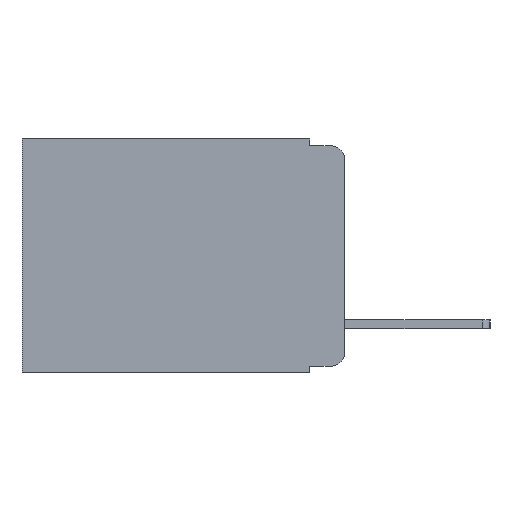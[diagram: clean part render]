
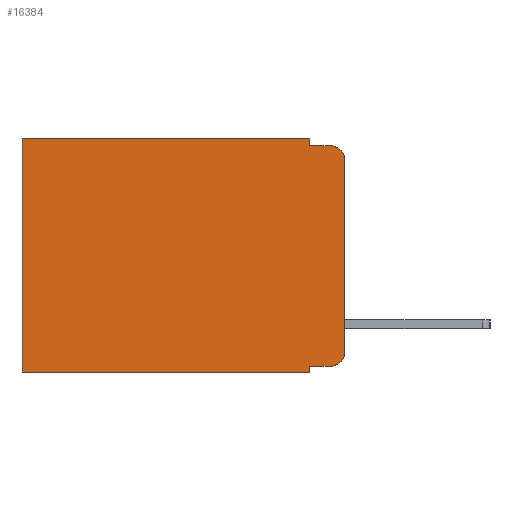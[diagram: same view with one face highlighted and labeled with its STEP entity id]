
A CAD part, left-side view. The second image highlights one B-rep face of the part: STEP entity #16384.
In plain terms, the highlighted planar face has unit normal (-1, 0, 0).
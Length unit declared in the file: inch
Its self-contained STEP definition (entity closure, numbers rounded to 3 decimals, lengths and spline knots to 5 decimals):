
#145 = ORIENTED_EDGE ( 'NONE', *, *, #16762, .F. ) ;
#662 = EDGE_CURVE ( 'NONE', #12113, #1314, #10611, .T. ) ;
#740 = CARTESIAN_POINT ( 'NONE',  ( 0.298, 0.051, -0.333 ) ) ;
#1314 = VERTEX_POINT ( 'NONE', #7506 ) ;
#1507 = DIRECTION ( 'NONE',  ( 0., 0., -1. ) ) ;
#2196 = CARTESIAN_POINT ( 'NONE',  ( 0.298, 0., -0.313 ) ) ;
#2331 = CIRCLE ( 'NONE', #8159, 0.02 ) ;
#2427 = VECTOR ( 'NONE', #5516, 39.37008 ) ;
#2864 = EDGE_CURVE ( 'NONE', #17752, #1314, #19845, .T. ) ;
#2885 = LINE ( 'NONE', #9695, #7057 ) ;
#3372 = AXIS2_PLACEMENT_3D ( 'NONE', #18085, #18155, #8942 ) ;
#3554 = LINE ( 'NONE', #16618, #7681 ) ;
#4242 = VECTOR ( 'NONE', #14819, 39.37008 ) ;
#4552 = VERTEX_POINT ( 'NONE', #19593 ) ;
#4815 = VERTEX_POINT ( 'NONE', #13018 ) ;
#5064 = DIRECTION ( 'NONE',  ( 0., 0., -1. ) ) ;
#5355 = VERTEX_POINT ( 'NONE', #2196 ) ;
#5516 = DIRECTION ( 'NONE',  ( 0., 1., 0. ) ) ;
#5737 = DIRECTION ( 'NONE',  ( 0., 0., -1. ) ) ;
#5811 = DIRECTION ( 'NONE',  ( 0., -1., 0. ) ) ;
#5813 = DIRECTION ( 'NONE',  ( 0., -1., 0. ) ) ;
#6029 = EDGE_CURVE ( 'NONE', #17752, #5355, #16909, .T. ) ;
#7057 = VECTOR ( 'NONE', #18810, 39.37008 ) ;
#7402 = PLANE ( 'NONE',  #3372 ) ;
#7426 = CARTESIAN_POINT ( 'NONE',  ( 0.298, 0.051, 0. ) ) ;
#7506 = CARTESIAN_POINT ( 'NONE',  ( 0.298, 0.02, -0.01 ) ) ;
#7681 = VECTOR ( 'NONE', #5813, 39.37008 ) ;
#8159 = AXIS2_PLACEMENT_3D ( 'NONE', #20023, #10915, #1507 ) ;
#8546 = CARTESIAN_POINT ( 'NONE',  ( 0.298, 0., -0.343 ) ) ;
#8942 = DIRECTION ( 'NONE',  ( 0., 0., -1. ) ) ;
#9107 = CARTESIAN_POINT ( 'NONE',  ( 0.298, 0.051, -0.01 ) ) ;
#9144 = CARTESIAN_POINT ( 'NONE',  ( 0.298, 0.051, -0.01 ) ) ;
#9329 = LINE ( 'NONE', #17887, #4242 ) ;
#9364 = ORIENTED_EDGE ( 'NONE', *, *, #14698, .T. ) ;
#9695 = CARTESIAN_POINT ( 'NONE',  ( 0.298, 0., 0. ) ) ;
#10480 = AXIS2_PLACEMENT_3D ( 'NONE', #18902, #11712, #13078 ) ;
#10611 = LINE ( 'NONE', #9107, #18732 ) ;
#10915 = DIRECTION ( 'NONE',  ( -1., 0., 0. ) ) ;
#11010 = VERTEX_POINT ( 'NONE', #13033 ) ;
#11119 = LINE ( 'NONE', #15153, #12104 ) ;
#11564 = FACE_OUTER_BOUND ( 'NONE', #17800, .T. ) ;
#11712 = DIRECTION ( 'NONE',  ( -1., 0., 0. ) ) ;
#11874 = EDGE_CURVE ( 'NONE', #11010, #4815, #14856, .T. ) ;
#11888 = ORIENTED_EDGE ( 'NONE', *, *, #2864, .T. ) ;
#12104 = VECTOR ( 'NONE', #16704, 39.37008 ) ;
#12113 = VERTEX_POINT ( 'NONE', #9144 ) ;
#12821 = CARTESIAN_POINT ( 'NONE',  ( 0.298, 0., 0. ) ) ;
#12844 = VECTOR ( 'NONE', #5064, 39.37008 ) ;
#13018 = CARTESIAN_POINT ( 'NONE',  ( 0.298, 0.473, -0.343 ) ) ;
#13033 = CARTESIAN_POINT ( 'NONE',  ( 0.298, 0.051, -0.343 ) ) ;
#13078 = DIRECTION ( 'NONE',  ( 0., 0., -1. ) ) ;
#13600 = ORIENTED_EDGE ( 'NONE', *, *, #18745, .T. ) ;
#13805 = ORIENTED_EDGE ( 'NONE', *, *, #14224, .T. ) ;
#14224 = EDGE_CURVE ( 'NONE', #17528, #16051, #2885, .T. ) ;
#14271 = CARTESIAN_POINT ( 'NONE',  ( 0.298, 0., -0.03 ) ) ;
#14698 = EDGE_CURVE ( 'NONE', #4552, #5355, #2331, .T. ) ;
#14819 = DIRECTION ( 'NONE',  ( 0., 0., -1. ) ) ;
#14856 = LINE ( 'NONE', #8546, #2427 ) ;
#15093 = ORIENTED_EDGE ( 'NONE', *, *, #11874, .F. ) ;
#15153 = CARTESIAN_POINT ( 'NONE',  ( 0.298, 0.473, 0. ) ) ;
#15751 = EDGE_CURVE ( 'NONE', #16275, #4552, #3554, .T. ) ;
#15918 = VECTOR ( 'NONE', #5737, 39.37008 ) ;
#16051 = VERTEX_POINT ( 'NONE', #17235 ) ;
#16275 = VERTEX_POINT ( 'NONE', #740 ) ;
#16383 = LINE ( 'NONE', #18110, #15918 ) ;
#16384 = ADVANCED_FACE ( 'NONE', ( #11564 ), #7402, .F. ) ;
#16618 = CARTESIAN_POINT ( 'NONE',  ( 0.298, 0.051, -0.333 ) ) ;
#16704 = DIRECTION ( 'NONE',  ( 0., 0., -1. ) ) ;
#16762 = EDGE_CURVE ( 'NONE', #16275, #11010, #9329, .T. ) ;
#16909 = LINE ( 'NONE', #12821, #12844 ) ;
#17235 = CARTESIAN_POINT ( 'NONE',  ( 0.298, 0.473, 0. ) ) ;
#17288 = ORIENTED_EDGE ( 'NONE', *, *, #6029, .F. ) ;
#17528 = VERTEX_POINT ( 'NONE', #7426 ) ;
#17752 = VERTEX_POINT ( 'NONE', #14271 ) ;
#17800 = EDGE_LOOP ( 'NONE', ( #17288, #11888, #18341, #18272, #13805, #13600, #15093, #145, #18285, #9364 ) ) ;
#17887 = CARTESIAN_POINT ( 'NONE',  ( 0.298, 0.051, 0. ) ) ;
#18085 = CARTESIAN_POINT ( 'NONE',  ( 0.298, 0., 0. ) ) ;
#18110 = CARTESIAN_POINT ( 'NONE',  ( 0.298, 0.051, 0. ) ) ;
#18155 = DIRECTION ( 'NONE',  ( 1., 0., 0. ) ) ;
#18272 = ORIENTED_EDGE ( 'NONE', *, *, #19746, .F. ) ;
#18285 = ORIENTED_EDGE ( 'NONE', *, *, #15751, .T. ) ;
#18341 = ORIENTED_EDGE ( 'NONE', *, *, #662, .F. ) ;
#18732 = VECTOR ( 'NONE', #5811, 39.37008 ) ;
#18745 = EDGE_CURVE ( 'NONE', #16051, #4815, #11119, .T. ) ;
#18810 = DIRECTION ( 'NONE',  ( 0., 1., 0. ) ) ;
#18902 = CARTESIAN_POINT ( 'NONE',  ( 0.298, 0.02, -0.03 ) ) ;
#19593 = CARTESIAN_POINT ( 'NONE',  ( 0.298, 0.02, -0.333 ) ) ;
#19746 = EDGE_CURVE ( 'NONE', #17528, #12113, #16383, .T. ) ;
#19845 = CIRCLE ( 'NONE', #10480, 0.02 ) ;
#20023 = CARTESIAN_POINT ( 'NONE',  ( 0.298, 0.02, -0.313 ) ) ;
